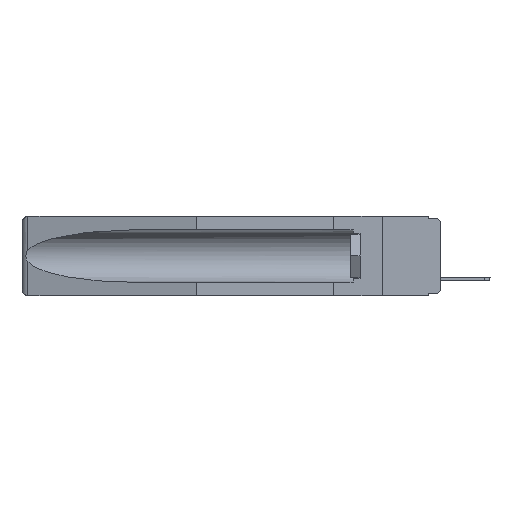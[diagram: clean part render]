
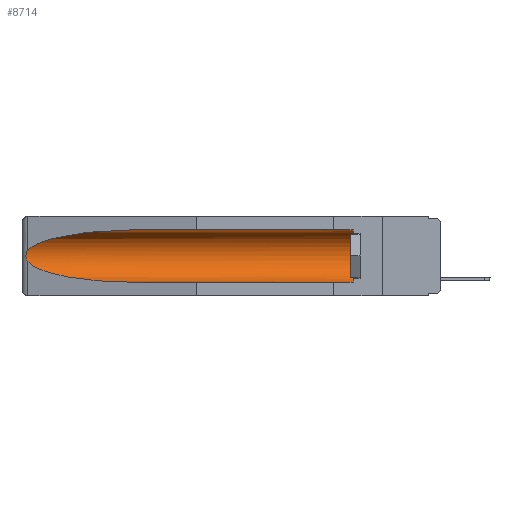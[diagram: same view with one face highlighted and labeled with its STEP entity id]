
A CAD part, left-side view. The second image highlights one B-rep face of the part: STEP entity #8714.
In plain terms, the highlighted cylindrical face has radius 2.857 mm (diameter 5.715 mm), a partial arc.
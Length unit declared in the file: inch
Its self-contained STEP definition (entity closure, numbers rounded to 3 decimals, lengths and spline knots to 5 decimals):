
#362 = VERTEX_POINT ( 'NONE', #684 ) ;
#489 = CARTESIAN_POINT ( 'NONE',  ( 0.26597, 1.5296, -0.19026 ) ) ;
#548 = CARTESIAN_POINT ( 'NONE',  ( 0.26654, 1.53092, -0.15636 ) ) ;
#684 = CARTESIAN_POINT ( 'NONE',  ( 0.26537, 1.52718, -0.19328 ) ) ;
#1696 = FACE_OUTER_BOUND ( 'NONE', #13049, .T. ) ;
#1953 = CARTESIAN_POINT ( 'NONE',  ( 0.26537, 1.52718, -0.19328 ) ) ;
#2100 = CARTESIAN_POINT ( 'NONE',  ( 0.155, 0.126, -0.284 ) ) ;
#2295 = EDGE_CURVE ( 'NONE', #10088, #362, #9892, .T. ) ;
#3339 = VECTOR ( 'NONE', #14120, 39.37008 ) ;
#3978 = LINE ( 'NONE', #16627, #3339 ) ;
#4230 = CARTESIAN_POINT ( 'NONE',  ( 0.25451, 1.48313, -0.09465 ) ) ;
#4271 = CARTESIAN_POINT ( 'NONE',  ( 0.155, 1.07973, -0.284 ) ) ;
#4437 = VERTEX_POINT ( 'NONE', #17107 ) ;
#4564 = CARTESIAN_POINT ( 'NONE',  ( 0.2675, 1.53308, -0.17534 ) ) ;
#4777 = ORIENTED_EDGE ( 'NONE', *, *, #11548, .T. ) ;
#4986 = EDGE_CURVE ( 'NONE', #6550, #4437, #3978, .T. ) ;
#5115 = VERTEX_POINT ( 'NONE', #13220 ) ;
#5391 = DIRECTION ( 'NONE',  ( 0., 1., 0. ) ) ;
#5578 = CYLINDRICAL_SURFACE ( 'NONE', #6761, 0.1125 ) ;
#5609 = CARTESIAN_POINT ( 'NONE',  ( 0.155, -0.30754, -0.1715 ) ) ;
#5777 = EDGE_CURVE ( 'NONE', #5115, #9504, #9336, .T. ) ;
#5888 = VECTOR ( 'NONE', #5391, 39.37008 ) ;
#6550 = VERTEX_POINT ( 'NONE', #2100 ) ;
#6642 = ORIENTED_EDGE ( 'NONE', *, *, #7017, .T. ) ;
#6687 = ORIENTED_EDGE ( 'NONE', *, *, #2295, .T. ) ;
#6720 = ORIENTED_EDGE ( 'NONE', *, *, #4986, .F. ) ;
#6760 = DIRECTION ( 'NONE',  ( 0., 0., 1. ) ) ;
#6761 = AXIS2_PLACEMENT_3D ( 'NONE', #5609, #15232, #6760 ) ;
#7017 = EDGE_CURVE ( 'NONE', #9504, #10088, #13882, .T. ) ;
#7200 = CARTESIAN_POINT ( 'NONE',  ( 0.26537, 1.52718, -0.14972 ) ) ;
#8473 = CARTESIAN_POINT ( 'NONE',  ( 0.21114, 1.30732, -0.284 ) ) ;
#8595 = CARTESIAN_POINT ( 'NONE',  ( 0.26655, 1.53094, -0.18657 ) ) ;
#8601 = DIRECTION ( 'NONE',  ( 0., -1., 0. ) ) ;
#8660 = CARTESIAN_POINT ( 'NONE',  ( 0.155, 0.126, -0.1715 ) ) ;
#8714 = ADVANCED_FACE ( 'NONE', ( #1696 ), #5578, .F. ) ;
#8770 = CARTESIAN_POINT ( 'NONE',  ( 0.26597, 1.52961, -0.15275 ) ) ;
#9306 = CARTESIAN_POINT ( 'NONE',  ( 0.26537, 1.52718, -0.14972 ) ) ;
#9336 = LINE ( 'NONE', #17839, #5888 ) ;
#9504 = VERTEX_POINT ( 'NONE', #16781 ) ;
#9518 = EDGE_CURVE ( 'NONE', #6550, #5115, #14179, .T. ) ;
#9892 = B_SPLINE_CURVE_WITH_KNOTS ( 'NONE', 3,
 ( #7200, #8770, #548, #15503, #14323, #4564, #12691, #8595, #489, #1953 ),
 .UNSPECIFIED., .F., .F.,
 ( 4, 2, 2, 2, 4 ),
 ( 0., 0.00029, 0.00058, 0.00087, 0.00117 ),
 .UNSPECIFIED. ) ;
#10088 = VERTEX_POINT ( 'NONE', #9306 ) ;
#11548 = EDGE_CURVE ( 'NONE', #362, #4437, #13419, .T. ) ;
#12691 = CARTESIAN_POINT ( 'NONE',  ( 0.2673, 1.53269, -0.17917 ) ) ;
#13049 = EDGE_LOOP ( 'NONE', ( #6642, #6687, #4777, #6720, #13460, #17694 ) ) ;
#13220 = CARTESIAN_POINT ( 'NONE',  ( 0.155, 0.126, -0.059 ) ) ;
#13235 = AXIS2_PLACEMENT_3D ( 'NONE', #8660, #8601, #15448 ) ;
#13419 =( BOUNDED_CURVE ( )  B_SPLINE_CURVE ( 3, ( #16543, #15216, #8473, #4271 ),
 .UNSPECIFIED., .F., .F. ) 
 B_SPLINE_CURVE_WITH_KNOTS ( ( 4, 4 ),
 ( 0.1948, 1.5708 ),
 .UNSPECIFIED. ) 
 CURVE ( )  GEOMETRIC_REPRESENTATION_ITEM ( )  RATIONAL_B_SPLINE_CURVE ( ( 1., 0.848, 0.848, 1. ) ) 
 REPRESENTATION_ITEM ( '' )  );
#13460 = ORIENTED_EDGE ( 'NONE', *, *, #9518, .T. ) ;
#13882 =( BOUNDED_CURVE ( )  B_SPLINE_CURVE ( 3, ( #15120, #13935, #4230, #13990 ),
 .UNSPECIFIED., .F., .F. ) 
 B_SPLINE_CURVE_WITH_KNOTS ( ( 4, 4 ),
 ( 4.71239, 6.08839 ),
 .UNSPECIFIED. ) 
 CURVE ( )  GEOMETRIC_REPRESENTATION_ITEM ( )  RATIONAL_B_SPLINE_CURVE ( ( 1., 0.848, 0.848, 1. ) ) 
 REPRESENTATION_ITEM ( '' )  );
#13935 = CARTESIAN_POINT ( 'NONE',  ( 0.21114, 1.30732, -0.059 ) ) ;
#13990 = CARTESIAN_POINT ( 'NONE',  ( 0.26537, 1.52718, -0.14972 ) ) ;
#14120 = DIRECTION ( 'NONE',  ( 0., 1., 0. ) ) ;
#14179 = CIRCLE ( 'NONE', #13235, 0.1125 ) ;
#14323 = CARTESIAN_POINT ( 'NONE',  ( 0.2675, 1.53308, -0.16763 ) ) ;
#15120 = CARTESIAN_POINT ( 'NONE',  ( 0.155, 1.07973, -0.059 ) ) ;
#15216 = CARTESIAN_POINT ( 'NONE',  ( 0.25451, 1.48313, -0.24835 ) ) ;
#15232 = DIRECTION ( 'NONE',  ( 0., 1., 0. ) ) ;
#15448 = DIRECTION ( 'NONE',  ( 0., 0., 1. ) ) ;
#15503 = CARTESIAN_POINT ( 'NONE',  ( 0.2673, 1.5327, -0.16383 ) ) ;
#16543 = CARTESIAN_POINT ( 'NONE',  ( 0.26537, 1.52718, -0.19328 ) ) ;
#16627 = CARTESIAN_POINT ( 'NONE',  ( 0.155, -0.30754, -0.284 ) ) ;
#16781 = CARTESIAN_POINT ( 'NONE',  ( 0.155, 1.07973, -0.059 ) ) ;
#17107 = CARTESIAN_POINT ( 'NONE',  ( 0.155, 1.07973, -0.284 ) ) ;
#17694 = ORIENTED_EDGE ( 'NONE', *, *, #5777, .T. ) ;
#17839 = CARTESIAN_POINT ( 'NONE',  ( 0.155, -0.30754, -0.059 ) ) ;
